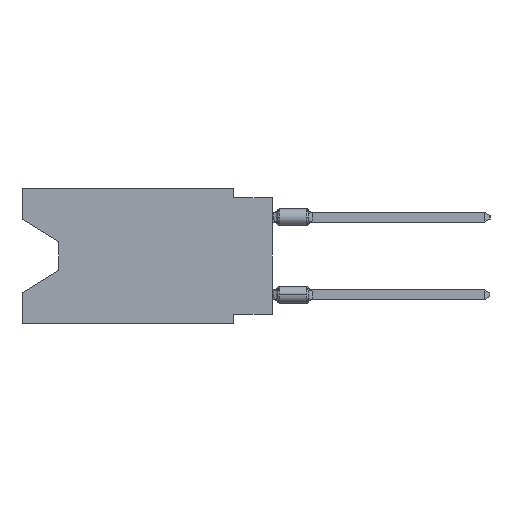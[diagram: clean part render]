
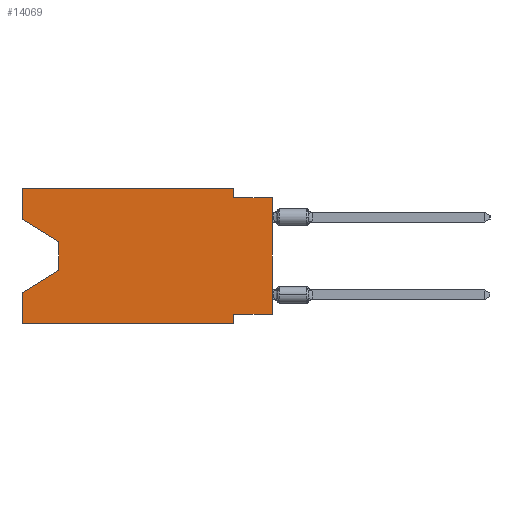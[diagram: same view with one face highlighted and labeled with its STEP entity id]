
A CAD part, left-side view. The second image highlights one B-rep face of the part: STEP entity #14069.
In plain terms, the highlighted planar face has unit normal (-1, 0, 0).
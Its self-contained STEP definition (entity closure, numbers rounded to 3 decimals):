
#97 = ORIENTED_EDGE ( 'NONE', *, *, #23016, .F. ) ;
#160 = VERTEX_POINT ( 'NONE', #8907 ) ;
#263 = LINE ( 'NONE', #21462, #23687 ) ;
#443 = DIRECTION ( 'NONE',  ( 0., -1., 0. ) ) ;
#685 = CARTESIAN_POINT ( 'NONE',  ( 0., 13.97, -5.385 ) ) ;
#767 = VECTOR ( 'NONE', #17463, 1000. ) ;
#771 = CARTESIAN_POINT ( 'NONE',  ( 0., 16.383, 0. ) ) ;
#1153 = LINE ( 'NONE', #15007, #24353 ) ;
#2106 = VECTOR ( 'NONE', #7722, 1000. ) ;
#2749 = DIRECTION ( 'NONE',  ( 0., 0.855, -0.519 ) ) ;
#2859 = EDGE_CURVE ( 'NONE', #18039, #5621, #29779, .T. ) ;
#3286 = CARTESIAN_POINT ( 'NONE',  ( 0., 0., -0.635 ) ) ;
#3672 = CARTESIAN_POINT ( 'NONE',  ( 0., 2.54, -0.635 ) ) ;
#3804 = CARTESIAN_POINT ( 'NONE',  ( 0., 2.54, -8.255 ) ) ;
#3948 = DIRECTION ( 'NONE',  ( 1., 0., 0. ) ) ;
#3957 = LINE ( 'NONE', #13537, #11336 ) ;
#4932 = VERTEX_POINT ( 'NONE', #6627 ) ;
#5374 = CARTESIAN_POINT ( 'NONE',  ( 0., 16.383, 0. ) ) ;
#5621 = VERTEX_POINT ( 'NONE', #17742 ) ;
#6627 = CARTESIAN_POINT ( 'NONE',  ( 0., 2.54, -8.89 ) ) ;
#7451 = CARTESIAN_POINT ( 'NONE',  ( 0., 16.383, -8.89 ) ) ;
#7722 = DIRECTION ( 'NONE',  ( 0., 0., 1. ) ) ;
#7867 = CARTESIAN_POINT ( 'NONE',  ( 0., 13.97, -3.505 ) ) ;
#7887 = LINE ( 'NONE', #5374, #767 ) ;
#7910 = EDGE_CURVE ( 'NONE', #23094, #19601, #7887, .T. ) ;
#8119 = ORIENTED_EDGE ( 'NONE', *, *, #25633, .F. ) ;
#8308 = DIRECTION ( 'NONE',  ( 0., -1., 0. ) ) ;
#8364 = ORIENTED_EDGE ( 'NONE', *, *, #2859, .F. ) ;
#8598 = VERTEX_POINT ( 'NONE', #29282 ) ;
#8785 = VECTOR ( 'NONE', #8308, 1000. ) ;
#8907 = CARTESIAN_POINT ( 'NONE',  ( 0., 13.97, -5.385 ) ) ;
#9075 = VERTEX_POINT ( 'NONE', #3804 ) ;
#10483 = EDGE_CURVE ( 'NONE', #9075, #4932, #3957, .T. ) ;
#11105 = EDGE_CURVE ( 'NONE', #16647, #23529, #21793, .T. ) ;
#11301 = CARTESIAN_POINT ( 'NONE',  ( 0., 0., -8.255 ) ) ;
#11336 = VECTOR ( 'NONE', #23086, 1000. ) ;
#11883 = ORIENTED_EDGE ( 'NONE', *, *, #11105, .F. ) ;
#11906 = EDGE_CURVE ( 'NONE', #19981, #5621, #14520, .T. ) ;
#12321 = DIRECTION ( 'NONE',  ( 0., 0., 1. ) ) ;
#12479 = AXIS2_PLACEMENT_3D ( 'NONE', #15889, #3948, #20730 ) ;
#13537 = CARTESIAN_POINT ( 'NONE',  ( 0., 2.54, -8.89 ) ) ;
#13675 = FACE_OUTER_BOUND ( 'NONE', #25056, .T. ) ;
#14069 = ADVANCED_FACE ( 'NONE', ( #13675 ), #18392, .F. ) ;
#14311 = VERTEX_POINT ( 'NONE', #7867 ) ;
#14520 = LINE ( 'NONE', #19386, #22144 ) ;
#14794 = EDGE_CURVE ( 'NONE', #8598, #14311, #1153, .T. ) ;
#14990 = ORIENTED_EDGE ( 'NONE', *, *, #29241, .T. ) ;
#15007 = CARTESIAN_POINT ( 'NONE',  ( 0., 16.383, -2.038 ) ) ;
#15889 = CARTESIAN_POINT ( 'NONE',  ( 0., 16.383, 0. ) ) ;
#16041 = CARTESIAN_POINT ( 'NONE',  ( 0., 16.383, -6.852 ) ) ;
#16411 = DIRECTION ( 'NONE',  ( 0., 1., 0. ) ) ;
#16647 = VERTEX_POINT ( 'NONE', #771 ) ;
#17463 = DIRECTION ( 'NONE',  ( 0., 0., 1. ) ) ;
#17494 = DIRECTION ( 'NONE',  ( 0., -1., 0. ) ) ;
#17742 = CARTESIAN_POINT ( 'NONE',  ( 0., 0., -0.635 ) ) ;
#17971 = EDGE_CURVE ( 'NONE', #23529, #18039, #27836, .T. ) ;
#18039 = VERTEX_POINT ( 'NONE', #3672 ) ;
#18135 = ORIENTED_EDGE ( 'NONE', *, *, #17971, .F. ) ;
#18392 = PLANE ( 'NONE',  #12479 ) ;
#18432 = DIRECTION ( 'NONE',  ( 0., 0., -1. ) ) ;
#18754 = LINE ( 'NONE', #7451, #30199 ) ;
#19386 = CARTESIAN_POINT ( 'NONE',  ( 0., 0., 0. ) ) ;
#19601 = VERTEX_POINT ( 'NONE', #16041 ) ;
#19654 = CARTESIAN_POINT ( 'NONE',  ( 0., 16.383, 0. ) ) ;
#19981 = VERTEX_POINT ( 'NONE', #11301 ) ;
#20382 = VECTOR ( 'NONE', #443, 1000. ) ;
#20730 = DIRECTION ( 'NONE',  ( 0., 0., -1. ) ) ;
#21246 = CARTESIAN_POINT ( 'NONE',  ( 0., 0., -8.255 ) ) ;
#21462 = CARTESIAN_POINT ( 'NONE',  ( 0., 13.97, -3.505 ) ) ;
#21793 = LINE ( 'NONE', #24301, #20382 ) ;
#22000 = LINE ( 'NONE', #19654, #2106 ) ;
#22144 = VECTOR ( 'NONE', #12321, 1000. ) ;
#22200 = DIRECTION ( 'NONE',  ( 0., -0.855, -0.519 ) ) ;
#22339 = CARTESIAN_POINT ( 'NONE',  ( 0., 16.383, -8.89 ) ) ;
#22729 = ORIENTED_EDGE ( 'NONE', *, *, #10483, .F. ) ;
#22853 = VECTOR ( 'NONE', #16411, 1000. ) ;
#23016 = EDGE_CURVE ( 'NONE', #19981, #9075, #30651, .T. ) ;
#23086 = DIRECTION ( 'NONE',  ( 0., 0., -1. ) ) ;
#23094 = VERTEX_POINT ( 'NONE', #22339 ) ;
#23529 = VERTEX_POINT ( 'NONE', #26690 ) ;
#23687 = VECTOR ( 'NONE', #24437, 1000. ) ;
#24301 = CARTESIAN_POINT ( 'NONE',  ( 0., 16.383, 0. ) ) ;
#24344 = EDGE_CURVE ( 'NONE', #23094, #4932, #18754, .T. ) ;
#24353 = VECTOR ( 'NONE', #22200, 1000. ) ;
#24437 = DIRECTION ( 'NONE',  ( 0., 0., -1. ) ) ;
#24724 = EDGE_CURVE ( 'NONE', #14311, #160, #263, .T. ) ;
#24867 = LINE ( 'NONE', #685, #25318 ) ;
#25056 = EDGE_LOOP ( 'NONE', ( #25484, #30060, #14990, #29415, #30223, #22729, #97, #25360, #8364, #18135, #11883, #8119 ) ) ;
#25168 = CARTESIAN_POINT ( 'NONE',  ( 0., 2.54, 0. ) ) ;
#25318 = VECTOR ( 'NONE', #2749, 1000. ) ;
#25360 = ORIENTED_EDGE ( 'NONE', *, *, #11906, .T. ) ;
#25484 = ORIENTED_EDGE ( 'NONE', *, *, #14794, .T. ) ;
#25633 = EDGE_CURVE ( 'NONE', #8598, #16647, #22000, .T. ) ;
#26215 = VECTOR ( 'NONE', #18432, 1000. ) ;
#26690 = CARTESIAN_POINT ( 'NONE',  ( 0., 2.54, 0. ) ) ;
#27836 = LINE ( 'NONE', #25168, #26215 ) ;
#29241 = EDGE_CURVE ( 'NONE', #160, #19601, #24867, .T. ) ;
#29282 = CARTESIAN_POINT ( 'NONE',  ( 0., 16.383, -2.038 ) ) ;
#29415 = ORIENTED_EDGE ( 'NONE', *, *, #7910, .F. ) ;
#29779 = LINE ( 'NONE', #3286, #8785 ) ;
#30060 = ORIENTED_EDGE ( 'NONE', *, *, #24724, .T. ) ;
#30199 = VECTOR ( 'NONE', #17494, 1000. ) ;
#30223 = ORIENTED_EDGE ( 'NONE', *, *, #24344, .T. ) ;
#30651 = LINE ( 'NONE', #21246, #22853 ) ;
